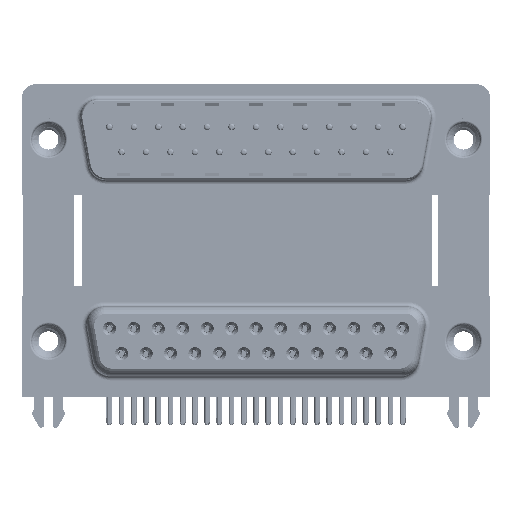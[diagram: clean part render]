
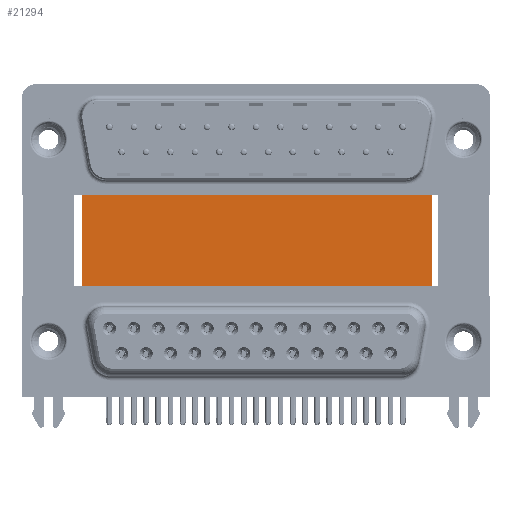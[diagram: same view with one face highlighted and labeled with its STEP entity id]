
A CAD part, top view. The second image highlights one B-rep face of the part: STEP entity #21294.
In plain terms, the highlighted planar face has unit normal (0, 0, 1).
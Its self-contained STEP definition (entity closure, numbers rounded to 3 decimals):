
#62 = VECTOR ( 'NONE', #15669, 1000. ) ;
#1644 = FACE_OUTER_BOUND ( 'NONE', #45926, .T. ) ;
#5849 = CARTESIAN_POINT ( 'NONE',  ( 3.79, -3.735, -12. ) ) ;
#6449 = LINE ( 'NONE', #39522, #45696 ) ;
#6799 = LINE ( 'NONE', #24271, #62 ) ;
#10537 = PLANE ( 'NONE',  #30406 ) ;
#13181 = ORIENTED_EDGE ( 'NONE', *, *, #28621, .F. ) ;
#15669 = DIRECTION ( 'NONE',  ( 0., -1., 0. ) ) ;
#15876 = ORIENTED_EDGE ( 'NONE', *, *, #53134, .T. ) ;
#16596 = VERTEX_POINT ( 'NONE', #5849 ) ;
#17125 = CARTESIAN_POINT ( 'NONE',  ( 3.79, 16.585, -12. ) ) ;
#20281 = EDGE_CURVE ( 'NONE', #24224, #47960, #6799, .T. ) ;
#21292 = VECTOR ( 'NONE', #56721, 1000. ) ;
#21294 = ADVANCED_FACE ( 'NONE', ( #1644 ), #10537, .F. ) ;
#23331 = DIRECTION ( 'NONE',  ( 0., -1., 0. ) ) ;
#24224 = VERTEX_POINT ( 'NONE', #41224 ) ;
#24271 = CARTESIAN_POINT ( 'NONE',  ( 43.43, 16.585, -12. ) ) ;
#27530 = VERTEX_POINT ( 'NONE', #33667 ) ;
#28021 = DIRECTION ( 'NONE',  ( -1., 0., 0. ) ) ;
#28621 = EDGE_CURVE ( 'NONE', #27530, #24224, #30583, .T. ) ;
#30406 = AXIS2_PLACEMENT_3D ( 'NONE', #50414, #54979, #28021 ) ;
#30583 = LINE ( 'NONE', #17125, #21292 ) ;
#30650 = DIRECTION ( 'NONE',  ( 1., 0., 0. ) ) ;
#30810 = VECTOR ( 'NONE', #23331, 1000. ) ;
#32061 = CARTESIAN_POINT ( 'NONE',  ( 43.43, -3.735, -12. ) ) ;
#33667 = CARTESIAN_POINT ( 'NONE',  ( 3.79, 16.585, -12. ) ) ;
#35428 = ORIENTED_EDGE ( 'NONE', *, *, #39625, .T. ) ;
#39522 = CARTESIAN_POINT ( 'NONE',  ( 3.79, -3.735, -12. ) ) ;
#39625 = EDGE_CURVE ( 'NONE', #16596, #47960, #6449, .T. ) ;
#41224 = CARTESIAN_POINT ( 'NONE',  ( 43.43, 16.585, -12. ) ) ;
#41664 = CARTESIAN_POINT ( 'NONE',  ( 3.79, 16.585, -12. ) ) ;
#45696 = VECTOR ( 'NONE', #30650, 1000. ) ;
#45926 = EDGE_LOOP ( 'NONE', ( #35428, #55078, #13181, #15876 ) ) ;
#46267 = LINE ( 'NONE', #41664, #30810 ) ;
#47960 = VERTEX_POINT ( 'NONE', #32061 ) ;
#50414 = CARTESIAN_POINT ( 'NONE',  ( 3.79, 16.585, -12. ) ) ;
#53134 = EDGE_CURVE ( 'NONE', #27530, #16596, #46267, .T. ) ;
#54979 = DIRECTION ( 'NONE',  ( 0., 0., -1. ) ) ;
#55078 = ORIENTED_EDGE ( 'NONE', *, *, #20281, .F. ) ;
#56721 = DIRECTION ( 'NONE',  ( 1., 0., 0. ) ) ;
